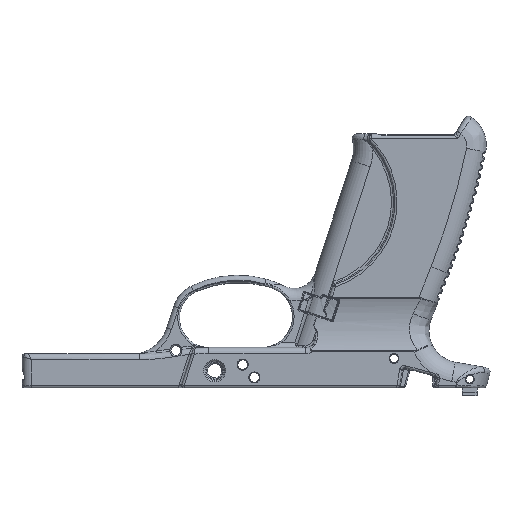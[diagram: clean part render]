
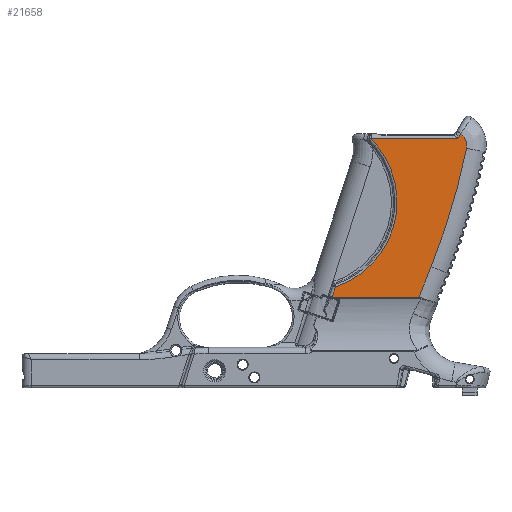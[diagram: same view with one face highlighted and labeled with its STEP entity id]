
A CAD part, front view. The second image highlights one B-rep face of the part: STEP entity #21658.
In plain terms, the highlighted planar face has unit normal (0, -1, 0).
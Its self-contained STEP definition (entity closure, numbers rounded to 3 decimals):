
#406=PLANE('',#23581);
#866=LINE('',#41075,#1970);
#1048=LINE('',#44862,#2152);
#1051=LINE('',#44885,#2155);
#1052=LINE('',#44888,#2156);
#1053=LINE('',#44892,#2157);
#1054=LINE('',#44894,#2158);
#1970=VECTOR('',#26685,10.);
#2152=VECTOR('',#27643,10.);
#2155=VECTOR('',#27656,10.);
#2156=VECTOR('',#27661,10.);
#2157=VECTOR('',#27664,10.);
#2158=VECTOR('',#27665,10.);
#3585=B_SPLINE_CURVE_WITH_KNOTS('',3,(#44896,#44897,#44898,#44899),
 .UNSPECIFIED.,.F.,.F.,(4,4),(0.,0.042),
 .UNSPECIFIED.);
#3586=B_SPLINE_CURVE_WITH_KNOTS('',3,(#44901,#44902,#44903,#44904),
 .UNSPECIFIED.,.F.,.F.,(4,4),(-0.882,-0.597),
 .UNSPECIFIED.);
#5016=FACE_OUTER_BOUND('',#6481,.T.);
#6481=EDGE_LOOP('',(#16820,#16821,#16822,#16823,#16824,#16825,#16826,#16827,
#16828,#16829,#16830));
#7653=CIRCLE('',#23047,282.274);
#7927=CIRCLE('',#23582,6.);
#7928=CIRCLE('',#23583,36.518);
#9207=VERTEX_POINT('',#36067);
#9208=VERTEX_POINT('',#36069);
#9321=VERTEX_POINT('',#41074);
#9646=VERTEX_POINT('',#44812);
#9647=VERTEX_POINT('',#44835);
#9653=VERTEX_POINT('',#44884);
#9654=VERTEX_POINT('',#44889);
#9655=VERTEX_POINT('',#44891);
#9656=VERTEX_POINT('',#44893);
#9657=VERTEX_POINT('',#44895);
#9658=VERTEX_POINT('',#44900);
#11386=EDGE_CURVE('',#9207,#9208,#7653,.T.);
#11610=EDGE_CURVE('',#9208,#9321,#866,.T.);
#12151=EDGE_CURVE('',#9647,#9646,#1048,.T.);
#12158=EDGE_CURVE('',#9646,#9653,#1051,.T.);
#12160=EDGE_CURVE('',#9321,#9647,#1052,.T.);
#12161=EDGE_CURVE('',#9654,#9207,#7927,.T.);
#12162=EDGE_CURVE('',#9655,#9654,#1053,.T.);
#12163=EDGE_CURVE('',#9656,#9655,#1054,.T.);
#12164=EDGE_CURVE('',#9657,#9656,#3585,.T.);
#12165=EDGE_CURVE('',#9658,#9657,#3586,.T.);
#12166=EDGE_CURVE('',#9653,#9658,#7928,.T.);
#16820=ORIENTED_EDGE('',*,*,#12151,.F.);
#16821=ORIENTED_EDGE('',*,*,#12160,.F.);
#16822=ORIENTED_EDGE('',*,*,#11610,.F.);
#16823=ORIENTED_EDGE('',*,*,#11386,.F.);
#16824=ORIENTED_EDGE('',*,*,#12161,.F.);
#16825=ORIENTED_EDGE('',*,*,#12162,.F.);
#16826=ORIENTED_EDGE('',*,*,#12163,.F.);
#16827=ORIENTED_EDGE('',*,*,#12164,.F.);
#16828=ORIENTED_EDGE('',*,*,#12165,.F.);
#16829=ORIENTED_EDGE('',*,*,#12166,.F.);
#16830=ORIENTED_EDGE('',*,*,#12158,.F.);
#21658=ADVANCED_FACE('',(#5016),#406,.T.);
#23047=AXIS2_PLACEMENT_3D('',#36070,#26345,#26346);
#23581=AXIS2_PLACEMENT_3D('',#44887,#27659,#27660);
#23582=AXIS2_PLACEMENT_3D('',#44890,#27662,#27663);
#23583=AXIS2_PLACEMENT_3D('',#44905,#27666,#27667);
#26345=DIRECTION('center_axis',(0.,1.,0.));
#26346=DIRECTION('ref_axis',(0.958,0.,-0.286));
#26685=DIRECTION('',(-0.371,0.,-0.929));
#27643=DIRECTION('',(-0.952,0.,0.306));
#27656=DIRECTION('',(0.309,0.,0.951));
#27659=DIRECTION('center_axis',(0.,-1.,0.));
#27660=DIRECTION('ref_axis',(1.,0.,0.));
#27661=DIRECTION('',(-1.,0.,0.));
#27662=DIRECTION('center_axis',(0.,1.,0.));
#27663=DIRECTION('ref_axis',(0.863,0.,0.505));
#27664=DIRECTION('',(0.531,0.,0.848));
#27665=DIRECTION('',(1.,0.,0.));
#27666=DIRECTION('center_axis',(0.,-1.,0.));
#27667=DIRECTION('ref_axis',(0.962,0.,-0.272));
#36067=CARTESIAN_POINT('',(89.046,-13.75,58.092));
#36069=CARTESIAN_POINT('',(74.571,-13.75,9.633));
#36070=CARTESIAN_POINT('Origin',(-187.57,-13.75,114.326));
#41074=CARTESIAN_POINT('',(69.538,-13.75,-2.968));
#41075=CARTESIAN_POINT('',(77.289,-13.75,16.44));
#44812=CARTESIAN_POINT('',(33.966,-13.75,-2.917));
#44835=CARTESIAN_POINT('',(34.127,-13.75,-2.968));
#44862=CARTESIAN_POINT('',(39.085,-13.75,-4.56));
#44884=CARTESIAN_POINT('',(35.343,-13.75,1.321));
#44885=CARTESIAN_POINT('',(35.678,-13.75,2.351));
#44887=CARTESIAN_POINT('Origin',(62.214,-13.75,30.354));
#44888=CARTESIAN_POINT('',(110.,-13.75,-2.968));
#44889=CARTESIAN_POINT('',(86.781,-13.75,64.076));
#44890=CARTESIAN_POINT('Origin',(83.166,-13.75,59.287));
#44891=CARTESIAN_POINT('',(85.482,-13.75,62.));
#44892=CARTESIAN_POINT('',(75.697,-13.75,46.369));
#44893=CARTESIAN_POINT('',(50.085,-13.75,62.));
#44894=CARTESIAN_POINT('',(51.607,-13.75,62.));
#44895=CARTESIAN_POINT('',(50.244,-13.75,61.619));
#44896=CARTESIAN_POINT('Ctrl Pts',(50.244,-13.75,61.619));
#44897=CARTESIAN_POINT('Ctrl Pts',(50.149,-13.75,61.723));
#44898=CARTESIAN_POINT('Ctrl Pts',(50.085,-13.75,61.859));
#44899=CARTESIAN_POINT('Ctrl Pts',(50.085,-13.75,62.));
#44900=CARTESIAN_POINT('',(52.112,-13.75,59.473));
#44901=CARTESIAN_POINT('Ctrl Pts',(52.112,-13.75,59.473));
#44902=CARTESIAN_POINT('Ctrl Pts',(51.504,-13.75,60.201));
#44903=CARTESIAN_POINT('Ctrl Pts',(50.881,-13.75,60.916));
#44904=CARTESIAN_POINT('Ctrl Pts',(50.244,-13.75,61.619));
#44905=CARTESIAN_POINT('Origin',(24.087,-13.75,36.061));
